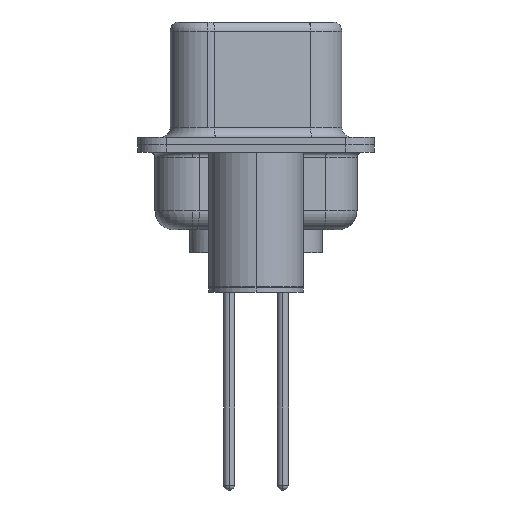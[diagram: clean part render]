
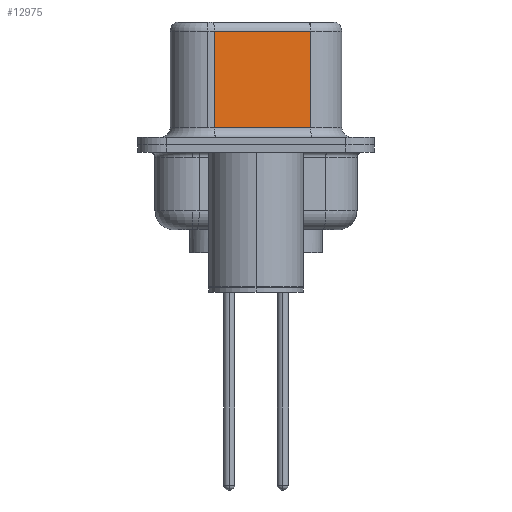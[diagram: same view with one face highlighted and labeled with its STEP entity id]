
A CAD part, left-side view. The second image highlights one B-rep face of the part: STEP entity #12975.
In plain terms, the highlighted planar face has unit normal (-0.985, -0.174, 0).
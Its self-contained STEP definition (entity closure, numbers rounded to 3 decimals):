
#157 = EDGE_LOOP ( 'NONE', ( #23117, #12024, #13777, #2037 ) ) ;
#483 = CARTESIAN_POINT ( 'NONE',  ( 4.58, -2.897, 6.52 ) ) ;
#1238 = CARTESIAN_POINT ( 'NONE',  ( 3.68, 2.203, 6.02 ) ) ;
#1294 = DIRECTION ( 'NONE',  ( -0.174, 0.985, 0. ) ) ;
#2037 = ORIENTED_EDGE ( 'NONE', *, *, #5007, .T. ) ;
#2291 = CARTESIAN_POINT ( 'NONE',  ( 4.58, -2.897, 6.52 ) ) ;
#4003 = DIRECTION ( 'NONE',  ( 0., 0., -1. ) ) ;
#4231 = PLANE ( 'NONE',  #6658 ) ;
#5007 = EDGE_CURVE ( 'NONE', #8736, #24797, #14562, .T. ) ;
#6658 = AXIS2_PLACEMENT_3D ( 'NONE', #2291, #14245, #22174 ) ;
#7285 = LINE ( 'NONE', #10926, #7896 ) ;
#7896 = VECTOR ( 'NONE', #1294, 1000. ) ;
#8394 = EDGE_CURVE ( 'NONE', #21788, #24797, #11936, .T. ) ;
#8736 = VERTEX_POINT ( 'NONE', #11777 ) ;
#9454 = CARTESIAN_POINT ( 'NONE',  ( 4.58, -2.897, 6.02 ) ) ;
#10926 = CARTESIAN_POINT ( 'NONE',  ( 4.58, -2.897, 6.02 ) ) ;
#11777 = CARTESIAN_POINT ( 'NONE',  ( 3.68, 2.203, 0.9 ) ) ;
#11786 = VECTOR ( 'NONE', #24568, 1000. ) ;
#11936 = LINE ( 'NONE', #483, #13534 ) ;
#12024 = ORIENTED_EDGE ( 'NONE', *, *, #15840, .T. ) ;
#12975 = ADVANCED_FACE ( 'NONE', ( #20098 ), #4231, .F. ) ;
#13534 = VECTOR ( 'NONE', #16089, 1000. ) ;
#13777 = ORIENTED_EDGE ( 'NONE', *, *, #17273, .T. ) ;
#13842 = CARTESIAN_POINT ( 'NONE',  ( 3.68, 2.203, 6.52 ) ) ;
#14245 = DIRECTION ( 'NONE',  ( 0.985, 0.174, 0. ) ) ;
#14562 = LINE ( 'NONE', #20417, #11786 ) ;
#15230 = CARTESIAN_POINT ( 'NONE',  ( 4.58, -2.897, 0.9 ) ) ;
#15840 = EDGE_CURVE ( 'NONE', #21788, #23584, #7285, .T. ) ;
#16089 = DIRECTION ( 'NONE',  ( 0., 0., -1. ) ) ;
#16269 = VECTOR ( 'NONE', #4003, 1000. ) ;
#17273 = EDGE_CURVE ( 'NONE', #23584, #8736, #17792, .T. ) ;
#17792 = LINE ( 'NONE', #13842, #16269 ) ;
#20098 = FACE_OUTER_BOUND ( 'NONE', #157, .T. ) ;
#20417 = CARTESIAN_POINT ( 'NONE',  ( 4.58, -2.897, 0.9 ) ) ;
#21788 = VERTEX_POINT ( 'NONE', #9454 ) ;
#22174 = DIRECTION ( 'NONE',  ( -0.174, 0.985, 0. ) ) ;
#23117 = ORIENTED_EDGE ( 'NONE', *, *, #8394, .F. ) ;
#23584 = VERTEX_POINT ( 'NONE', #1238 ) ;
#24568 = DIRECTION ( 'NONE',  ( 0.174, -0.985, 0. ) ) ;
#24797 = VERTEX_POINT ( 'NONE', #15230 ) ;
